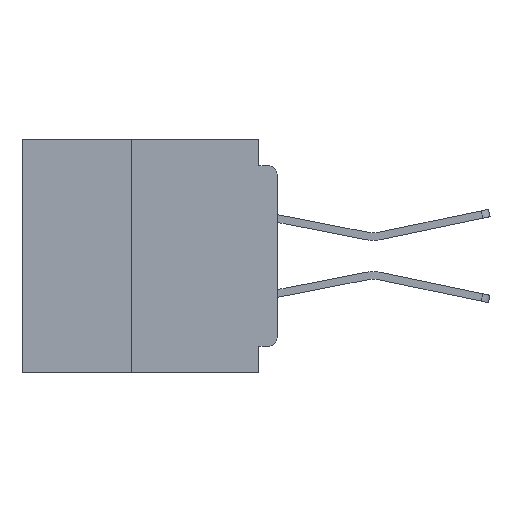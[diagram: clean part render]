
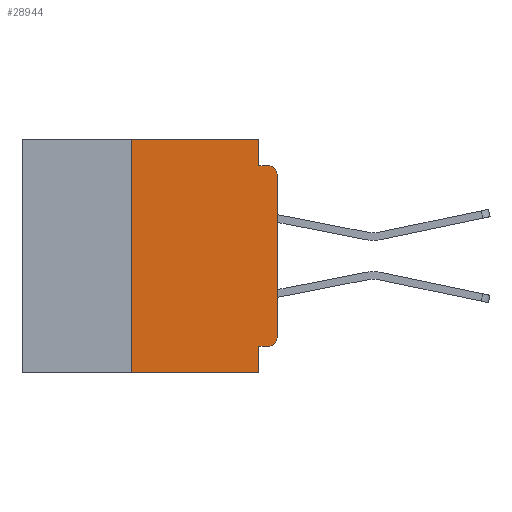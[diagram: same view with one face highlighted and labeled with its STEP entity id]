
A CAD part, left-side view. The second image highlights one B-rep face of the part: STEP entity #28944.
In plain terms, the highlighted planar face has unit normal (-1, 0, 0).
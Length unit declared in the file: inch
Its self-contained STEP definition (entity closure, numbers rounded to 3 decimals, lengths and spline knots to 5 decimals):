
#1559 = ORIENTED_EDGE ( 'NONE', *, *, #10116, .F. ) ;
#1563 = EDGE_CURVE ( 'NONE', #35635, #33028, #20999, .T. ) ;
#2058 = VERTEX_POINT ( 'NONE', #37178 ) ;
#2073 = CARTESIAN_POINT ( 'NONE',  ( 0., 0., -0.355 ) ) ;
#2537 = EDGE_LOOP ( 'NONE', ( #34444, #18516, #1559, #26121, #36167, #5186, #14902, #24815, #15753, #26060 ) ) ;
#2672 = AXIS2_PLACEMENT_3D ( 'NONE', #26331, #8597, #29275 ) ;
#3105 = VERTEX_POINT ( 'NONE', #27234 ) ;
#5186 = ORIENTED_EDGE ( 'NONE', *, *, #25894, .F. ) ;
#7713 = VECTOR ( 'NONE', #19189, 39.37008 ) ;
#7995 = EDGE_CURVE ( 'NONE', #23878, #25672, #36774, .T. ) ;
#8597 = DIRECTION ( 'NONE',  ( -1., 0., 0. ) ) ;
#8642 = VERTEX_POINT ( 'NONE', #27382 ) ;
#8955 = EDGE_CURVE ( 'NONE', #23878, #2058, #25353, .T. ) ;
#9733 = CARTESIAN_POINT ( 'NONE',  ( 0., 0.437, 0. ) ) ;
#10116 = EDGE_CURVE ( 'NONE', #8642, #33028, #23465, .T. ) ;
#10344 = LINE ( 'NONE', #26909, #32904 ) ;
#11064 = CARTESIAN_POINT ( 'NONE',  ( 0., 0.437, -0.4 ) ) ;
#11975 = EDGE_CURVE ( 'NONE', #32575, #8642, #25715, .T. ) ;
#12745 = DIRECTION ( 'NONE',  ( 0., 0., -1. ) ) ;
#13239 = LINE ( 'NONE', #27694, #35699 ) ;
#13968 = CARTESIAN_POINT ( 'NONE',  ( 0., 0., -0.06 ) ) ;
#14317 = CARTESIAN_POINT ( 'NONE',  ( 0., 0.031, 0. ) ) ;
#14902 = ORIENTED_EDGE ( 'NONE', *, *, #35675, .T. ) ;
#15219 = DIRECTION ( 'NONE',  ( -1., 0., 0. ) ) ;
#15251 = CARTESIAN_POINT ( 'NONE',  ( 0., 0.015, -0.045 ) ) ;
#15753 = ORIENTED_EDGE ( 'NONE', *, *, #8955, .F. ) ;
#16669 = AXIS2_PLACEMENT_3D ( 'NONE', #9733, #30393, #12745 ) ;
#17778 = AXIS2_PLACEMENT_3D ( 'NONE', #32762, #15219, #35681 ) ;
#17936 = CARTESIAN_POINT ( 'NONE',  ( 0., 0.25, -0.4 ) ) ;
#18516 = ORIENTED_EDGE ( 'NONE', *, *, #1563, .T. ) ;
#18797 = VECTOR ( 'NONE', #29001, 39.37008 ) ;
#19189 = DIRECTION ( 'NONE',  ( 0., -1., 0. ) ) ;
#20999 = CIRCLE ( 'NONE', #2672, 0.015 ) ;
#22864 = DIRECTION ( 'NONE',  ( 0., 1., 0. ) ) ;
#22919 = VECTOR ( 'NONE', #28972, 39.37008 ) ;
#22927 = FACE_OUTER_BOUND ( 'NONE', #2537, .T. ) ;
#23205 = CARTESIAN_POINT ( 'NONE',  ( 0., 0.031, -0.4 ) ) ;
#23465 = LINE ( 'NONE', #25094, #7713 ) ;
#23878 = VERTEX_POINT ( 'NONE', #30309 ) ;
#24068 = DIRECTION ( 'NONE',  ( 0., 0., 1. ) ) ;
#24290 = VERTEX_POINT ( 'NONE', #23205 ) ;
#24478 = PLANE ( 'NONE',  #16669 ) ;
#24815 = ORIENTED_EDGE ( 'NONE', *, *, #35722, .F. ) ;
#24921 = CARTESIAN_POINT ( 'NONE',  ( 0., 0.031, 0. ) ) ;
#25094 = CARTESIAN_POINT ( 'NONE',  ( 0., 0., -0.045 ) ) ;
#25353 = LINE ( 'NONE', #2073, #33091 ) ;
#25672 = VERTEX_POINT ( 'NONE', #34574 ) ;
#25715 = LINE ( 'NONE', #14317, #22919 ) ;
#25894 = EDGE_CURVE ( 'NONE', #26997, #3105, #26991, .T. ) ;
#25934 = EDGE_CURVE ( 'NONE', #25672, #35635, #10344, .T. ) ;
#26050 = CARTESIAN_POINT ( 'NONE',  ( 0., 0.031, -0.4 ) ) ;
#26060 = ORIENTED_EDGE ( 'NONE', *, *, #7995, .T. ) ;
#26121 = ORIENTED_EDGE ( 'NONE', *, *, #11975, .F. ) ;
#26331 = CARTESIAN_POINT ( 'NONE',  ( 0., 0.015, -0.06 ) ) ;
#26909 = CARTESIAN_POINT ( 'NONE',  ( 0., 0., 0. ) ) ;
#26991 = LINE ( 'NONE', #17936, #33819 ) ;
#26997 = VERTEX_POINT ( 'NONE', #38069 ) ;
#27234 = CARTESIAN_POINT ( 'NONE',  ( 0., 0.25, 0. ) ) ;
#27382 = CARTESIAN_POINT ( 'NONE',  ( 0., 0.031, -0.045 ) ) ;
#27694 = CARTESIAN_POINT ( 'NONE',  ( 0., 0.437, 0. ) ) ;
#28474 = LINE ( 'NONE', #11064, #35259 ) ;
#28944 = ADVANCED_FACE ( 'NONE', ( #22927 ), #24478, .F. ) ;
#28972 = DIRECTION ( 'NONE',  ( 0., 0., -1. ) ) ;
#29001 = DIRECTION ( 'NONE',  ( 0., 0., -1. ) ) ;
#29015 = EDGE_CURVE ( 'NONE', #3105, #32575, #13239, .T. ) ;
#29275 = DIRECTION ( 'NONE',  ( 0., 0., -1. ) ) ;
#30309 = CARTESIAN_POINT ( 'NONE',  ( 0., 0.015, -0.355 ) ) ;
#30393 = DIRECTION ( 'NONE',  ( 1., 0., 0. ) ) ;
#30753 = DIRECTION ( 'NONE',  ( 0., -1., 0. ) ) ;
#32575 = VERTEX_POINT ( 'NONE', #24921 ) ;
#32644 = DIRECTION ( 'NONE',  ( 0., 0., 1. ) ) ;
#32762 = CARTESIAN_POINT ( 'NONE',  ( 0., 0.015, -0.34 ) ) ;
#32904 = VECTOR ( 'NONE', #24068, 39.37008 ) ;
#33028 = VERTEX_POINT ( 'NONE', #15251 ) ;
#33091 = VECTOR ( 'NONE', #22864, 39.37008 ) ;
#33819 = VECTOR ( 'NONE', #32644, 39.37008 ) ;
#34361 = LINE ( 'NONE', #26050, #18797 ) ;
#34444 = ORIENTED_EDGE ( 'NONE', *, *, #25934, .T. ) ;
#34574 = CARTESIAN_POINT ( 'NONE',  ( 0., 0., -0.34 ) ) ;
#34589 = DIRECTION ( 'NONE',  ( 0., -1., 0. ) ) ;
#35259 = VECTOR ( 'NONE', #34589, 39.37008 ) ;
#35635 = VERTEX_POINT ( 'NONE', #13968 ) ;
#35675 = EDGE_CURVE ( 'NONE', #26997, #24290, #28474, .T. ) ;
#35681 = DIRECTION ( 'NONE',  ( 0., 0., -1. ) ) ;
#35699 = VECTOR ( 'NONE', #30753, 39.37008 ) ;
#35722 = EDGE_CURVE ( 'NONE', #2058, #24290, #34361, .T. ) ;
#36167 = ORIENTED_EDGE ( 'NONE', *, *, #29015, .F. ) ;
#36774 = CIRCLE ( 'NONE', #17778, 0.015 ) ;
#37178 = CARTESIAN_POINT ( 'NONE',  ( 0., 0.031, -0.355 ) ) ;
#38069 = CARTESIAN_POINT ( 'NONE',  ( 0., 0.25, -0.4 ) ) ;
